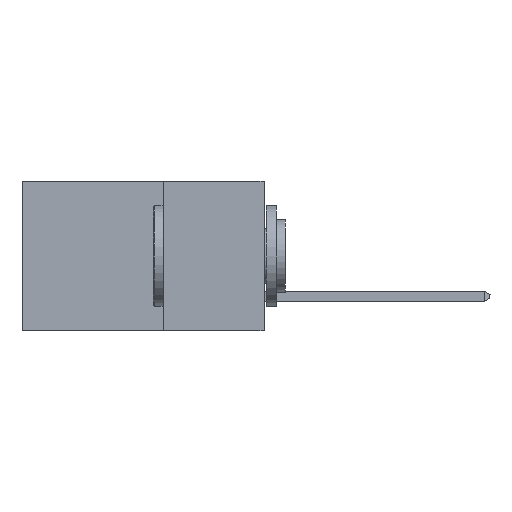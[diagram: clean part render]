
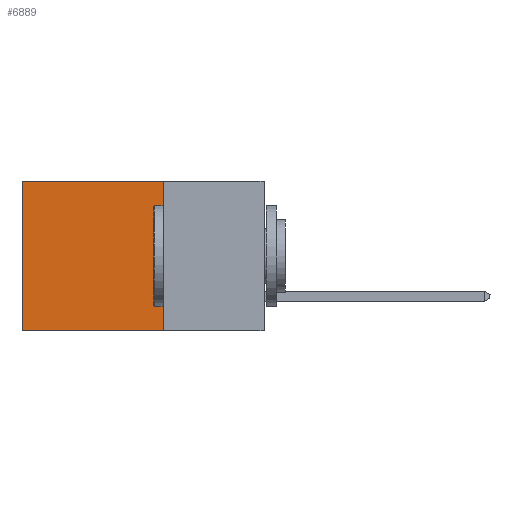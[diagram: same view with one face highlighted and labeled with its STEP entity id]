
A CAD part, left-side view. The second image highlights one B-rep face of the part: STEP entity #6889.
In plain terms, the highlighted planar face has unit normal (-1, 0, 0).
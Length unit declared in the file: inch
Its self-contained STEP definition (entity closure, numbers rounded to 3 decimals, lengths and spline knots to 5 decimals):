
#78 = CARTESIAN_POINT ( 'NONE',  ( 0.2615, 0.25, 0. ) ) ;
#179 = CARTESIAN_POINT ( 'NONE',  ( 0.2615, 0.6, -0.37 ) ) ;
#510 = DIRECTION ( 'NONE',  ( 0., 1., 0. ) ) ;
#779 = ORIENTED_EDGE ( 'NONE', *, *, #20647, .F. ) ;
#1660 = VERTEX_POINT ( 'NONE', #78 ) ;
#3087 = DIRECTION ( 'NONE',  ( 0., 0., -1. ) ) ;
#4305 = DIRECTION ( 'NONE',  ( 0., 1., 0. ) ) ;
#4315 = EDGE_CURVE ( 'NONE', #1660, #13108, #22022, .T. ) ;
#4546 = VECTOR ( 'NONE', #23277, 39.37008 ) ;
#4869 = VECTOR ( 'NONE', #510, 39.37008 ) ;
#4940 = LINE ( 'NONE', #14342, #24437 ) ;
#5325 = CARTESIAN_POINT ( 'NONE',  ( 0.2615, 0.25, 0. ) ) ;
#6180 = CARTESIAN_POINT ( 'NONE',  ( 0.2615, 0.6, -0.37 ) ) ;
#6522 = AXIS2_PLACEMENT_3D ( 'NONE', #23935, #23785, #23761 ) ;
#6889 = ADVANCED_FACE ( 'NONE', ( #19494 ), #23791, .F. ) ;
#8842 = EDGE_CURVE ( 'NONE', #1660, #12397, #4940, .T. ) ;
#11775 = CARTESIAN_POINT ( 'NONE',  ( 0.2615, 0.25, -0.37 ) ) ;
#11878 = VECTOR ( 'NONE', #4305, 39.37008 ) ;
#12397 = VERTEX_POINT ( 'NONE', #19185 ) ;
#13108 = VERTEX_POINT ( 'NONE', #17680 ) ;
#14045 = EDGE_LOOP ( 'NONE', ( #16903, #779, #21029, #23506 ) ) ;
#14342 = CARTESIAN_POINT ( 'NONE',  ( 0.2615, 0.25, -0.37 ) ) ;
#14997 = LINE ( 'NONE', #11775, #4869 ) ;
#16903 = ORIENTED_EDGE ( 'NONE', *, *, #21366, .T. ) ;
#17680 = CARTESIAN_POINT ( 'NONE',  ( 0.2615, 0.6, 0. ) ) ;
#19094 = LINE ( 'NONE', #6180, #4546 ) ;
#19185 = CARTESIAN_POINT ( 'NONE',  ( 0.2615, 0.25, -0.37 ) ) ;
#19494 = FACE_OUTER_BOUND ( 'NONE', #14045, .T. ) ;
#20525 = VERTEX_POINT ( 'NONE', #179 ) ;
#20647 = EDGE_CURVE ( 'NONE', #12397, #20525, #14997, .T. ) ;
#21029 = ORIENTED_EDGE ( 'NONE', *, *, #8842, .F. ) ;
#21366 = EDGE_CURVE ( 'NONE', #13108, #20525, #19094, .T. ) ;
#22022 = LINE ( 'NONE', #5325, #11878 ) ;
#23277 = DIRECTION ( 'NONE',  ( 0., 0., -1. ) ) ;
#23506 = ORIENTED_EDGE ( 'NONE', *, *, #4315, .T. ) ;
#23761 = DIRECTION ( 'NONE',  ( 0., 0., -1. ) ) ;
#23785 = DIRECTION ( 'NONE',  ( 1., 0., 0. ) ) ;
#23791 = PLANE ( 'NONE',  #6522 ) ;
#23935 = CARTESIAN_POINT ( 'NONE',  ( 0.2615, 0.25, -0.37 ) ) ;
#24437 = VECTOR ( 'NONE', #3087, 39.37008 ) ;
